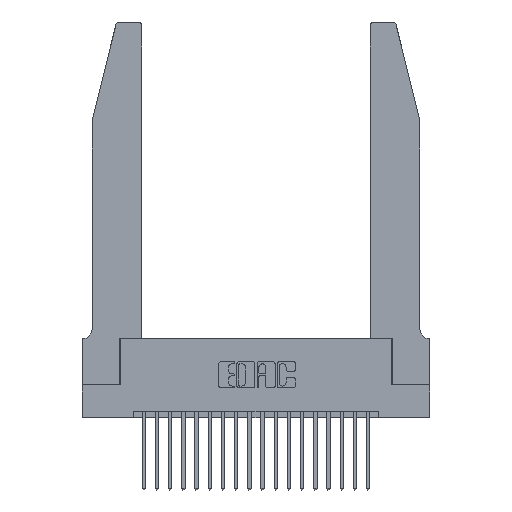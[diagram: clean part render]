
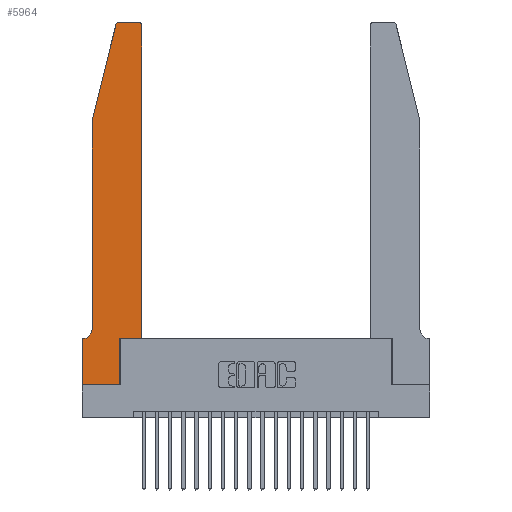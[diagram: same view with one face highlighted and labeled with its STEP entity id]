
A CAD part, top view. The second image highlights one B-rep face of the part: STEP entity #5964.
In plain terms, the highlighted planar face has unit normal (0, 0, 1).
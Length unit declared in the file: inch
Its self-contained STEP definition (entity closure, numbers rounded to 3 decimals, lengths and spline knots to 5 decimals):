
#42 = ORIENTED_EDGE ( 'NONE', *, *, #20874, .T. ) ;
#170 = DIRECTION ( 'NONE',  ( 1., 0., 0. ) ) ;
#472 = DIRECTION ( 'NONE',  ( 0., 1., 0. ) ) ;
#622 = AXIS2_PLACEMENT_3D ( 'NONE', #19285, #14011, #15655 ) ;
#989 = VECTOR ( 'NONE', #19318, 39.37008 ) ;
#1547 = CIRCLE ( 'NONE', #8733, 0.03 ) ;
#1556 = DIRECTION ( 'NONE',  ( 1., 0., 0. ) ) ;
#1595 = AXIS2_PLACEMENT_3D ( 'NONE', #3813, #17498, #19234 ) ;
#1656 = DIRECTION ( 'NONE',  ( 0., 0., 1. ) ) ;
#1802 = EDGE_CURVE ( 'NONE', #4568, #16862, #7217, .T. ) ;
#2239 = CARTESIAN_POINT ( 'NONE',  ( 0.4505, 2.72, 0.37 ) ) ;
#2623 = VERTEX_POINT ( 'NONE', #13964 ) ;
#2685 = CARTESIAN_POINT ( 'NONE',  ( 0.4505, 0.35, 0.37 ) ) ;
#3107 = CARTESIAN_POINT ( 'NONE',  ( 0.4205, 2.75, 0.37 ) ) ;
#3407 = VERTEX_POINT ( 'NONE', #22091 ) ;
#3609 = EDGE_CURVE ( 'NONE', #9212, #10875, #13852, .T. ) ;
#3736 = CARTESIAN_POINT ( 'NONE',  ( 0.4505, 0.35, 0.37 ) ) ;
#3807 = LINE ( 'NONE', #14610, #9490 ) ;
#3813 = CARTESIAN_POINT ( 'NONE',  ( 0.0055, 0.42, 0.37 ) ) ;
#3957 = VECTOR ( 'NONE', #472, 39.37008 ) ;
#4087 = ORIENTED_EDGE ( 'NONE', *, *, #9126, .T. ) ;
#4136 = VECTOR ( 'NONE', #4816, 39.37008 ) ;
#4528 = ORIENTED_EDGE ( 'NONE', *, *, #7450, .T. ) ;
#4568 = VERTEX_POINT ( 'NONE', #3107 ) ;
#4720 = VECTOR ( 'NONE', #1556, 39.37008 ) ;
#4816 = DIRECTION ( 'NONE',  ( 0., 1., 0. ) ) ;
#5099 = DIRECTION ( 'NONE',  ( 0., -1., 0. ) ) ;
#5179 = CARTESIAN_POINT ( 'NONE',  ( 0.4505, 0.35, 0.37 ) ) ;
#5297 = ORIENTED_EDGE ( 'NONE', *, *, #17016, .T. ) ;
#5760 = ORIENTED_EDGE ( 'NONE', *, *, #21494, .T. ) ;
#5964 = ADVANCED_FACE ( 'NONE', ( #11769 ), #10102, .T. ) ;
#6096 = CARTESIAN_POINT ( 'NONE',  ( 0.2865, 0.35, 0.37 ) ) ;
#6433 = ORIENTED_EDGE ( 'NONE', *, *, #3609, .T. ) ;
#7034 = DIRECTION ( 'NONE',  ( 1., 0., 0. ) ) ;
#7184 = CARTESIAN_POINT ( 'NONE',  ( 0., 0., 0.37 ) ) ;
#7217 = LINE ( 'NONE', #10849, #989 ) ;
#7279 = DIRECTION ( 'NONE',  ( 1., 0., 0. ) ) ;
#7450 = EDGE_CURVE ( 'NONE', #10875, #11040, #16196, .T. ) ;
#7606 = VERTEX_POINT ( 'NONE', #14950 ) ;
#7845 = EDGE_CURVE ( 'NONE', #11040, #4568, #21212, .T. ) ;
#8353 = CARTESIAN_POINT ( 'NONE',  ( 0.0755, 0.35, 0.37 ) ) ;
#8733 = AXIS2_PLACEMENT_3D ( 'NONE', #13780, #15489, #7279 ) ;
#9126 = EDGE_CURVE ( 'NONE', #20540, #14238, #10267, .T. ) ;
#9212 = VERTEX_POINT ( 'NONE', #6096 ) ;
#9255 = DIRECTION ( 'NONE',  ( -0.239, -0.971, 0. ) ) ;
#9325 = EDGE_CURVE ( 'NONE', #15247, #2623, #16915, .T. ) ;
#9490 = VECTOR ( 'NONE', #19882, 39.37008 ) ;
#10102 = PLANE ( 'NONE',  #20791 ) ;
#10267 = LINE ( 'NONE', #12775, #21960 ) ;
#10849 = CARTESIAN_POINT ( 'NONE',  ( 0.2605, 2.75, 0.37 ) ) ;
#10875 = VERTEX_POINT ( 'NONE', #3736 ) ;
#11040 = VERTEX_POINT ( 'NONE', #2239 ) ;
#11143 = CARTESIAN_POINT ( 'NONE',  ( 0.0055, 0.35, 0.37 ) ) ;
#11280 = CARTESIAN_POINT ( 'NONE',  ( 0., 0., 0.37 ) ) ;
#11769 = FACE_OUTER_BOUND ( 'NONE', #20013, .T. ) ;
#11952 = VERTEX_POINT ( 'NONE', #11280 ) ;
#12230 = LINE ( 'NONE', #20378, #21747 ) ;
#12419 = VECTOR ( 'NONE', #13437, 39.37008 ) ;
#12775 = CARTESIAN_POINT ( 'NONE',  ( 0.0755, 2., 0.37 ) ) ;
#13437 = DIRECTION ( 'NONE',  ( -1., 0., 0. ) ) ;
#13541 = ORIENTED_EDGE ( 'NONE', *, *, #16313, .T. ) ;
#13780 = CARTESIAN_POINT ( 'NONE',  ( 0.284, 2.72, 0.37 ) ) ;
#13852 = LINE ( 'NONE', #5179, #4720 ) ;
#13964 = CARTESIAN_POINT ( 'NONE',  ( 0., 0.35, 0.37 ) ) ;
#14011 = DIRECTION ( 'NONE',  ( 0., 0., 1. ) ) ;
#14238 = VERTEX_POINT ( 'NONE', #15698 ) ;
#14514 = ORIENTED_EDGE ( 'NONE', *, *, #17710, .T. ) ;
#14610 = CARTESIAN_POINT ( 'NONE',  ( 0., 0., 0.37 ) ) ;
#14950 = CARTESIAN_POINT ( 'NONE',  ( 0.0755, 0.42, 0.37 ) ) ;
#15226 = ORIENTED_EDGE ( 'NONE', *, *, #7845, .T. ) ;
#15247 = VERTEX_POINT ( 'NONE', #11143 ) ;
#15249 = CARTESIAN_POINT ( 'NONE',  ( 0., 0.35, 0.37 ) ) ;
#15489 = DIRECTION ( 'NONE',  ( 0., 0., 1. ) ) ;
#15655 = DIRECTION ( 'NONE',  ( 1., 0., 0. ) ) ;
#15698 = CARTESIAN_POINT ( 'NONE',  ( 0.0755, 2., 0.37 ) ) ;
#16196 = LINE ( 'NONE', #2685, #4136 ) ;
#16232 = CARTESIAN_POINT ( 'NONE',  ( 0.25487, 2.72718, 0.37 ) ) ;
#16312 = LINE ( 'NONE', #21094, #3957 ) ;
#16313 = EDGE_CURVE ( 'NONE', #2623, #11952, #3807, .T. ) ;
#16730 = ORIENTED_EDGE ( 'NONE', *, *, #21064, .T. ) ;
#16862 = VERTEX_POINT ( 'NONE', #17351 ) ;
#16915 = LINE ( 'NONE', #8353, #12419 ) ;
#17016 = EDGE_CURVE ( 'NONE', #7606, #15247, #21672, .T. ) ;
#17351 = CARTESIAN_POINT ( 'NONE',  ( 0.284, 2.75, 0.37 ) ) ;
#17498 = DIRECTION ( 'NONE',  ( 0., 0., -1. ) ) ;
#17710 = EDGE_CURVE ( 'NONE', #14238, #7606, #12230, .T. ) ;
#18510 = ORIENTED_EDGE ( 'NONE', *, *, #9325, .T. ) ;
#19234 = DIRECTION ( 'NONE',  ( -1., 0., 0. ) ) ;
#19285 = CARTESIAN_POINT ( 'NONE',  ( 0.4205, 2.72, 0.37 ) ) ;
#19297 = ORIENTED_EDGE ( 'NONE', *, *, #1802, .T. ) ;
#19318 = DIRECTION ( 'NONE',  ( -1., 0., 0. ) ) ;
#19491 = LINE ( 'NONE', #7184, #20257 ) ;
#19882 = DIRECTION ( 'NONE',  ( 0., -1., 0. ) ) ;
#20013 = EDGE_LOOP ( 'NONE', ( #19297, #42, #4087, #14514, #5297, #18510, #13541, #5760, #16730, #6433, #4528, #15226 ) ) ;
#20257 = VECTOR ( 'NONE', #170, 39.37008 ) ;
#20378 = CARTESIAN_POINT ( 'NONE',  ( 0.0755, 2., 0.37 ) ) ;
#20540 = VERTEX_POINT ( 'NONE', #16232 ) ;
#20791 = AXIS2_PLACEMENT_3D ( 'NONE', #15249, #1656, #7034 ) ;
#20874 = EDGE_CURVE ( 'NONE', #16862, #20540, #1547, .T. ) ;
#21064 = EDGE_CURVE ( 'NONE', #3407, #9212, #16312, .T. ) ;
#21094 = CARTESIAN_POINT ( 'NONE',  ( 0.2865, 0.35, 0.37 ) ) ;
#21212 = CIRCLE ( 'NONE', #622, 0.03 ) ;
#21494 = EDGE_CURVE ( 'NONE', #11952, #3407, #19491, .T. ) ;
#21672 = CIRCLE ( 'NONE', #1595, 0.07 ) ;
#21747 = VECTOR ( 'NONE', #5099, 39.37008 ) ;
#21960 = VECTOR ( 'NONE', #9255, 39.37008 ) ;
#22091 = CARTESIAN_POINT ( 'NONE',  ( 0.2865, 0., 0.37 ) ) ;
